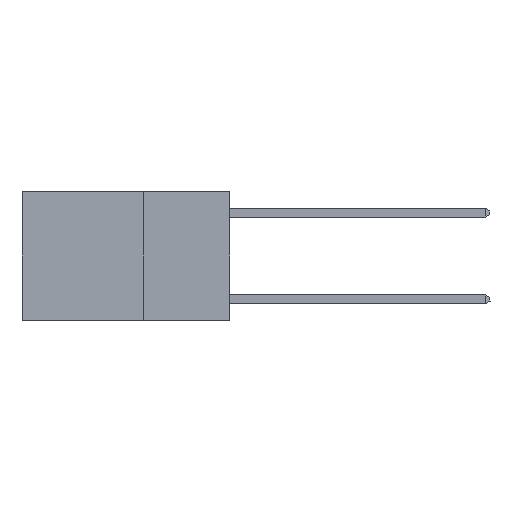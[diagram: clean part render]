
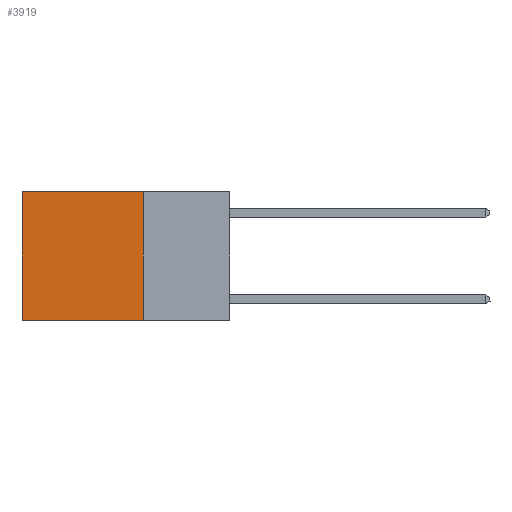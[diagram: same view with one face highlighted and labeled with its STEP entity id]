
A CAD part, left-side view. The second image highlights one B-rep face of the part: STEP entity #3919.
In plain terms, the highlighted planar face has unit normal (-1, 0, 0).
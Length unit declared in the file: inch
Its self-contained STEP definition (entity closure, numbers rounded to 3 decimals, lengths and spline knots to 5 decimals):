
#426 = CARTESIAN_POINT ( 'NONE',  ( 0.2625, 0.6, 0. ) ) ;
#436 = VERTEX_POINT ( 'NONE', #5653 ) ;
#1518 = EDGE_CURVE ( 'NONE', #3626, #436, #1614, .T. ) ;
#1535 = EDGE_LOOP ( 'NONE', ( #1956, #14316, #2881, #3353 ) ) ;
#1542 = VECTOR ( 'NONE', #7248, 39.37008 ) ;
#1614 = LINE ( 'NONE', #18445, #8631 ) ;
#1956 = ORIENTED_EDGE ( 'NONE', *, *, #10028, .T. ) ;
#2534 = EDGE_CURVE ( 'NONE', #11552, #9140, #13247, .T. ) ;
#2881 = ORIENTED_EDGE ( 'NONE', *, *, #16796, .F. ) ;
#2920 = FACE_OUTER_BOUND ( 'NONE', #1535, .T. ) ;
#3353 = ORIENTED_EDGE ( 'NONE', *, *, #1518, .T. ) ;
#3626 = VERTEX_POINT ( 'NONE', #12468 ) ;
#3919 = ADVANCED_FACE ( 'NONE', ( #2920 ), #8903, .F. ) ;
#4392 = CARTESIAN_POINT ( 'NONE',  ( 0.2625, 0.25, 0. ) ) ;
#4449 = DIRECTION ( 'NONE',  ( 0., 0., -1. ) ) ;
#5653 = CARTESIAN_POINT ( 'NONE',  ( 0.2625, 0.6, 0. ) ) ;
#6385 = DIRECTION ( 'NONE',  ( 0., 0., -1. ) ) ;
#6992 = CARTESIAN_POINT ( 'NONE',  ( 0.2625, 0.25, -0.37 ) ) ;
#7248 = DIRECTION ( 'NONE',  ( 0., 0., -1. ) ) ;
#8631 = VECTOR ( 'NONE', #15441, 39.37008 ) ;
#8903 = PLANE ( 'NONE',  #14951 ) ;
#9140 = VERTEX_POINT ( 'NONE', #14615 ) ;
#9299 = VECTOR ( 'NONE', #12978, 39.37008 ) ;
#10028 = EDGE_CURVE ( 'NONE', #436, #9140, #12382, .T. ) ;
#11552 = VERTEX_POINT ( 'NONE', #19199 ) ;
#12382 = LINE ( 'NONE', #426, #16382 ) ;
#12468 = CARTESIAN_POINT ( 'NONE',  ( 0.2625, 0.25, 0. ) ) ;
#12978 = DIRECTION ( 'NONE',  ( 0., 1., 0. ) ) ;
#13247 = LINE ( 'NONE', #6992, #9299 ) ;
#13372 = DIRECTION ( 'NONE',  ( 1., 0., 0. ) ) ;
#14316 = ORIENTED_EDGE ( 'NONE', *, *, #2534, .F. ) ;
#14615 = CARTESIAN_POINT ( 'NONE',  ( 0.2625, 0.6, -0.37 ) ) ;
#14672 = CARTESIAN_POINT ( 'NONE',  ( 0.2625, 0.25, 0. ) ) ;
#14951 = AXIS2_PLACEMENT_3D ( 'NONE', #4392, #13372, #4449 ) ;
#15441 = DIRECTION ( 'NONE',  ( 0., 1., 0. ) ) ;
#16382 = VECTOR ( 'NONE', #6385, 39.37008 ) ;
#16796 = EDGE_CURVE ( 'NONE', #3626, #11552, #17444, .T. ) ;
#17444 = LINE ( 'NONE', #14672, #1542 ) ;
#18445 = CARTESIAN_POINT ( 'NONE',  ( 0.2625, 0.25, 0. ) ) ;
#19199 = CARTESIAN_POINT ( 'NONE',  ( 0.2625, 0.25, -0.37 ) ) ;
